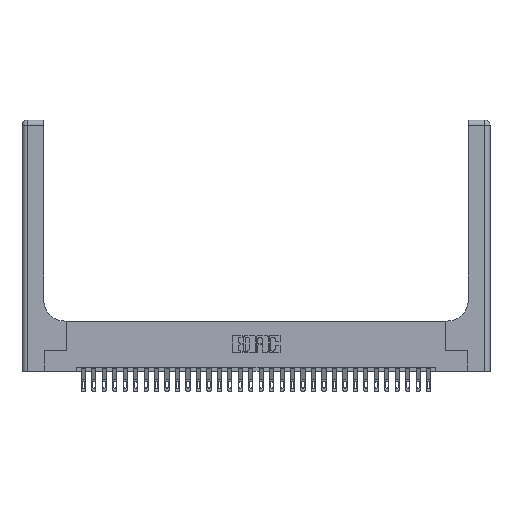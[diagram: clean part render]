
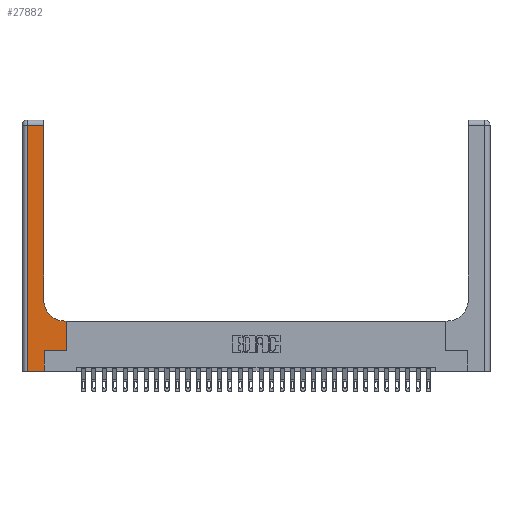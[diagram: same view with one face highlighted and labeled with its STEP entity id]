
A CAD part, top view. The second image highlights one B-rep face of the part: STEP entity #27882.
In plain terms, the highlighted planar face has unit normal (0, 0, 1).
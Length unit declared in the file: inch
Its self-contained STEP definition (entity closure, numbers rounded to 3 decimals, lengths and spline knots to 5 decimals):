
#473 = EDGE_CURVE ( 'NONE', #26046, #10242, #24746, .T. ) ;
#898 = ORIENTED_EDGE ( 'NONE', *, *, #10199, .T. ) ;
#1226 = LINE ( 'NONE', #19314, #24140 ) ;
#1818 = ORIENTED_EDGE ( 'NONE', *, *, #19035, .T. ) ;
#2107 = AXIS2_PLACEMENT_3D ( 'NONE', #21689, #17369, #8405 ) ;
#2240 = VECTOR ( 'NONE', #11952, 39.37008 ) ;
#2634 = ORIENTED_EDGE ( 'NONE', *, *, #19502, .T. ) ;
#2749 = VERTEX_POINT ( 'NONE', #22433 ) ;
#4043 = FACE_OUTER_BOUND ( 'NONE', #16087, .T. ) ;
#4849 = CARTESIAN_POINT ( 'NONE',  ( 0.26, 2.94, 0.37 ) ) ;
#4937 = DIRECTION ( 'NONE',  ( 0., 0., -1. ) ) ;
#6564 = VECTOR ( 'NONE', #28631, 39.37008 ) ;
#6663 = AXIS2_PLACEMENT_3D ( 'NONE', #7075, #4937, #24729 ) ;
#7075 = CARTESIAN_POINT ( 'NONE',  ( 0.51, 0.85, 0.37 ) ) ;
#7215 = CARTESIAN_POINT ( 'NONE',  ( 0.06, 0., 0.37 ) ) ;
#7444 = VERTEX_POINT ( 'NONE', #10433 ) ;
#7859 = EDGE_CURVE ( 'NONE', #2749, #7444, #25958, .T. ) ;
#7891 = DIRECTION ( 'NONE',  ( 1., 0., 0. ) ) ;
#8238 = EDGE_CURVE ( 'NONE', #10242, #22109, #19650, .T. ) ;
#8405 = DIRECTION ( 'NONE',  ( -1., 0., 0. ) ) ;
#8596 = PLANE ( 'NONE',  #2107 ) ;
#8653 = VERTEX_POINT ( 'NONE', #7215 ) ;
#9265 = ORIENTED_EDGE ( 'NONE', *, *, #17436, .T. ) ;
#9925 = VERTEX_POINT ( 'NONE', #28142 ) ;
#10199 = EDGE_CURVE ( 'NONE', #7444, #27441, #17419, .T. ) ;
#10242 = VERTEX_POINT ( 'NONE', #10477 ) ;
#10433 = CARTESIAN_POINT ( 'NONE',  ( 0.26, 0.85, 0.37 ) ) ;
#10434 = CARTESIAN_POINT ( 'NONE',  ( 0.265, 0., 0.37 ) ) ;
#10477 = CARTESIAN_POINT ( 'NONE',  ( 0.265, 0.25, 0.37 ) ) ;
#11525 = VECTOR ( 'NONE', #24760, 39.37008 ) ;
#11952 = DIRECTION ( 'NONE',  ( -1., 0., 0. ) ) ;
#12018 = CARTESIAN_POINT ( 'NONE',  ( 0.265, 0.25, 0.37 ) ) ;
#12388 = LINE ( 'NONE', #26391, #6564 ) ;
#13036 = VECTOR ( 'NONE', #7891, 39.37008 ) ;
#13042 = CARTESIAN_POINT ( 'NONE',  ( 0., 2.94, 0.37 ) ) ;
#14088 = VERTEX_POINT ( 'NONE', #23942 ) ;
#14393 = ORIENTED_EDGE ( 'NONE', *, *, #24092, .T. ) ;
#14765 = CARTESIAN_POINT ( 'NONE',  ( 0.265, 0., 0.37 ) ) ;
#14820 = ORIENTED_EDGE ( 'NONE', *, *, #473, .T. ) ;
#14946 = DIRECTION ( 'NONE',  ( 1., 0., 0. ) ) ;
#16087 = EDGE_LOOP ( 'NONE', ( #898, #2634, #14393, #1818, #14820, #26961, #16465, #9265, #28697 ) ) ;
#16465 = ORIENTED_EDGE ( 'NONE', *, *, #16835, .T. ) ;
#16835 = EDGE_CURVE ( 'NONE', #22109, #14088, #12388, .T. ) ;
#17204 = LINE ( 'NONE', #18147, #20360 ) ;
#17369 = DIRECTION ( 'NONE',  ( 0., 0., -1. ) ) ;
#17419 = LINE ( 'NONE', #22322, #11525 ) ;
#17436 = EDGE_CURVE ( 'NONE', #14088, #2749, #17204, .T. ) ;
#18147 = CARTESIAN_POINT ( 'NONE',  ( 0.26, 0.6, 0.37 ) ) ;
#19035 = EDGE_CURVE ( 'NONE', #8653, #26046, #1226, .T. ) ;
#19314 = CARTESIAN_POINT ( 'NONE',  ( 0., 0., 0.37 ) ) ;
#19502 = EDGE_CURVE ( 'NONE', #27441, #9925, #20620, .T. ) ;
#19650 = LINE ( 'NONE', #12018, #13036 ) ;
#20360 = VECTOR ( 'NONE', #22647, 39.37008 ) ;
#20620 = LINE ( 'NONE', #13042, #2240 ) ;
#20753 = CARTESIAN_POINT ( 'NONE',  ( 0.528, 0.25, 0.37 ) ) ;
#21689 = CARTESIAN_POINT ( 'NONE',  ( 0., 3., 0.37 ) ) ;
#22109 = VERTEX_POINT ( 'NONE', #20753 ) ;
#22254 = LINE ( 'NONE', #27894, #26469 ) ;
#22322 = CARTESIAN_POINT ( 'NONE',  ( 0.26, 3., 0.37 ) ) ;
#22433 = CARTESIAN_POINT ( 'NONE',  ( 0.51, 0.6, 0.37 ) ) ;
#22647 = DIRECTION ( 'NONE',  ( -1., 0., 0. ) ) ;
#23942 = CARTESIAN_POINT ( 'NONE',  ( 0.528, 0.6, 0.37 ) ) ;
#24092 = EDGE_CURVE ( 'NONE', #9925, #8653, #22254, .T. ) ;
#24140 = VECTOR ( 'NONE', #14946, 39.37008 ) ;
#24729 = DIRECTION ( 'NONE',  ( 1., 0., 0. ) ) ;
#24746 = LINE ( 'NONE', #14765, #28591 ) ;
#24760 = DIRECTION ( 'NONE',  ( 0., 1., 0. ) ) ;
#25958 = CIRCLE ( 'NONE', #6663, 0.25 ) ;
#26008 = DIRECTION ( 'NONE',  ( 0., 1., 0. ) ) ;
#26046 = VERTEX_POINT ( 'NONE', #10434 ) ;
#26391 = CARTESIAN_POINT ( 'NONE',  ( 0.528, 0.25, 0.37 ) ) ;
#26469 = VECTOR ( 'NONE', #27622, 39.37008 ) ;
#26961 = ORIENTED_EDGE ( 'NONE', *, *, #8238, .T. ) ;
#27441 = VERTEX_POINT ( 'NONE', #4849 ) ;
#27622 = DIRECTION ( 'NONE',  ( 0., -1., 0. ) ) ;
#27882 = ADVANCED_FACE ( 'NONE', ( #4043 ), #8596, .F. ) ;
#27894 = CARTESIAN_POINT ( 'NONE',  ( 0.06, 3., 0.37 ) ) ;
#28142 = CARTESIAN_POINT ( 'NONE',  ( 0.06, 2.94, 0.37 ) ) ;
#28591 = VECTOR ( 'NONE', #26008, 39.37008 ) ;
#28631 = DIRECTION ( 'NONE',  ( 0., 1., 0. ) ) ;
#28697 = ORIENTED_EDGE ( 'NONE', *, *, #7859, .T. ) ;
